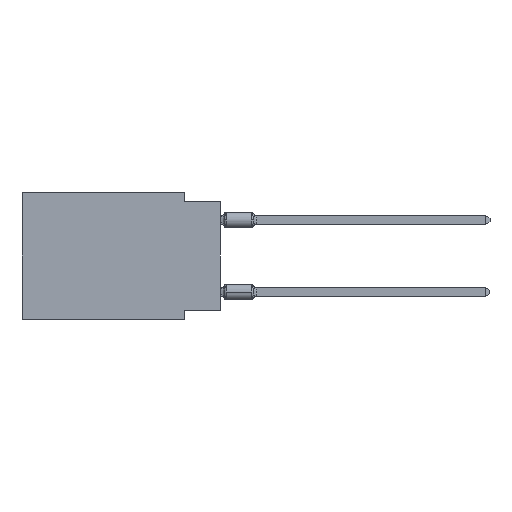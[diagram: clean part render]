
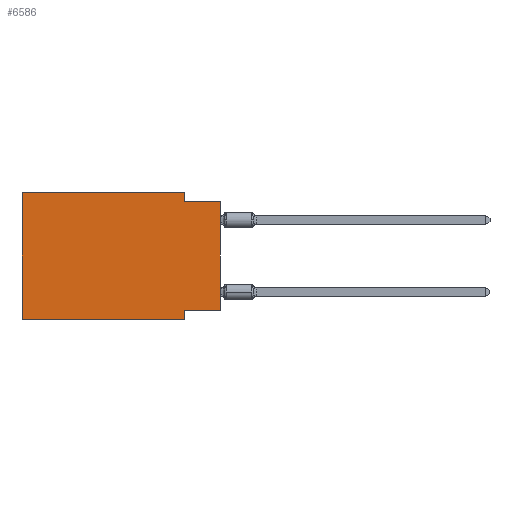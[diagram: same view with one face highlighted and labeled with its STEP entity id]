
A CAD part, left-side view. The second image highlights one B-rep face of the part: STEP entity #6586.
In plain terms, the highlighted planar face has unit normal (-1, 0, 0).
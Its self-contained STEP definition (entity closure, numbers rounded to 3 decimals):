
#11 = LINE ( 'NONE', #26151, #9679 ) ;
#76 = DIRECTION ( 'NONE',  ( 0., 0., -1. ) ) ;
#133 = DIRECTION ( 'NONE',  ( 0., 0., 1. ) ) ;
#521 = LINE ( 'NONE', #25059, #21888 ) ;
#904 = DIRECTION ( 'NONE',  ( 0., -1., 0. ) ) ;
#1095 = EDGE_CURVE ( 'NONE', #21548, #26164, #25565, .T. ) ;
#1410 = CARTESIAN_POINT ( 'NONE',  ( 0., 0., -8.255 ) ) ;
#1932 = CARTESIAN_POINT ( 'NONE',  ( 0., 13.97, 0. ) ) ;
#2087 = CARTESIAN_POINT ( 'NONE',  ( 0., 13.97, 0. ) ) ;
#2169 = CARTESIAN_POINT ( 'NONE',  ( 0., 2.54, -8.255 ) ) ;
#2215 = VERTEX_POINT ( 'NONE', #1932 ) ;
#2284 = VERTEX_POINT ( 'NONE', #2870 ) ;
#2870 = CARTESIAN_POINT ( 'NONE',  ( 0., 2.54, -0.635 ) ) ;
#2966 = DIRECTION ( 'NONE',  ( 0., -1., 0. ) ) ;
#3191 = CARTESIAN_POINT ( 'NONE',  ( 0., 13.97, 0. ) ) ;
#3408 = CARTESIAN_POINT ( 'NONE',  ( 0., 2.54, -8.89 ) ) ;
#3535 = AXIS2_PLACEMENT_3D ( 'NONE', #2087, #12183, #76 ) ;
#4265 = DIRECTION ( 'NONE',  ( 0., -1., 0. ) ) ;
#4320 = EDGE_LOOP ( 'NONE', ( #15920, #16107, #10689, #15969, #14798, #8347, #8427, #13978 ) ) ;
#4564 = VECTOR ( 'NONE', #19690, 1000. ) ;
#4584 = EDGE_CURVE ( 'NONE', #21560, #26164, #12329, .T. ) ;
#6586 = ADVANCED_FACE ( 'NONE', ( #13768 ), #23819, .F. ) ;
#6952 = LINE ( 'NONE', #22873, #16251 ) ;
#7720 = CARTESIAN_POINT ( 'NONE',  ( 0., 0., -8.255 ) ) ;
#8325 = VECTOR ( 'NONE', #14330, 1000. ) ;
#8347 = ORIENTED_EDGE ( 'NONE', *, *, #1095, .T. ) ;
#8427 = ORIENTED_EDGE ( 'NONE', *, *, #4584, .F. ) ;
#9679 = VECTOR ( 'NONE', #133, 1000. ) ;
#9761 = CARTESIAN_POINT ( 'NONE',  ( 0., 2.54, 0. ) ) ;
#10635 = EDGE_CURVE ( 'NONE', #2215, #15349, #521, .T. ) ;
#10689 = ORIENTED_EDGE ( 'NONE', *, *, #11133, .F. ) ;
#10758 = EDGE_CURVE ( 'NONE', #21548, #2215, #25591, .T. ) ;
#11133 = EDGE_CURVE ( 'NONE', #15349, #2284, #19823, .T. ) ;
#11673 = EDGE_CURVE ( 'NONE', #19404, #25139, #11, .T. ) ;
#12183 = DIRECTION ( 'NONE',  ( 1., 0., 0. ) ) ;
#12329 = LINE ( 'NONE', #19880, #8325 ) ;
#13455 = DIRECTION ( 'NONE',  ( 0., 1., 0. ) ) ;
#13768 = FACE_OUTER_BOUND ( 'NONE', #4320, .T. ) ;
#13978 = ORIENTED_EDGE ( 'NONE', *, *, #21683, .F. ) ;
#14330 = DIRECTION ( 'NONE',  ( 0., 0., -1. ) ) ;
#14798 = ORIENTED_EDGE ( 'NONE', *, *, #10758, .F. ) ;
#15349 = VERTEX_POINT ( 'NONE', #19314 ) ;
#15920 = ORIENTED_EDGE ( 'NONE', *, *, #11673, .T. ) ;
#15969 = ORIENTED_EDGE ( 'NONE', *, *, #10635, .F. ) ;
#16107 = ORIENTED_EDGE ( 'NONE', *, *, #16923, .F. ) ;
#16251 = VECTOR ( 'NONE', #2966, 1000. ) ;
#16923 = EDGE_CURVE ( 'NONE', #2284, #25139, #6952, .T. ) ;
#18726 = CARTESIAN_POINT ( 'NONE',  ( 0., 0., -0.635 ) ) ;
#19314 = CARTESIAN_POINT ( 'NONE',  ( 0., 2.54, 0. ) ) ;
#19404 = VERTEX_POINT ( 'NONE', #1410 ) ;
#19690 = DIRECTION ( 'NONE',  ( 0., 0., -1. ) ) ;
#19823 = LINE ( 'NONE', #9761, #4564 ) ;
#19880 = CARTESIAN_POINT ( 'NONE',  ( 0., 2.54, -8.89 ) ) ;
#21094 = VECTOR ( 'NONE', #13455, 1000. ) ;
#21325 = CARTESIAN_POINT ( 'NONE',  ( 0., 13.97, -8.89 ) ) ;
#21380 = VECTOR ( 'NONE', #904, 1000. ) ;
#21548 = VERTEX_POINT ( 'NONE', #22351 ) ;
#21560 = VERTEX_POINT ( 'NONE', #2169 ) ;
#21683 = EDGE_CURVE ( 'NONE', #19404, #21560, #25878, .T. ) ;
#21888 = VECTOR ( 'NONE', #4265, 1000. ) ;
#22351 = CARTESIAN_POINT ( 'NONE',  ( 0., 13.97, -8.89 ) ) ;
#22873 = CARTESIAN_POINT ( 'NONE',  ( 0., 0., -0.635 ) ) ;
#23215 = DIRECTION ( 'NONE',  ( 0., 0., 1. ) ) ;
#23819 = PLANE ( 'NONE',  #3535 ) ;
#24451 = VECTOR ( 'NONE', #23215, 1000. ) ;
#25059 = CARTESIAN_POINT ( 'NONE',  ( 0., 13.97, 0. ) ) ;
#25139 = VERTEX_POINT ( 'NONE', #18726 ) ;
#25565 = LINE ( 'NONE', #21325, #21380 ) ;
#25591 = LINE ( 'NONE', #3191, #24451 ) ;
#25878 = LINE ( 'NONE', #7720, #21094 ) ;
#26151 = CARTESIAN_POINT ( 'NONE',  ( 0., 0., 0. ) ) ;
#26164 = VERTEX_POINT ( 'NONE', #3408 ) ;
